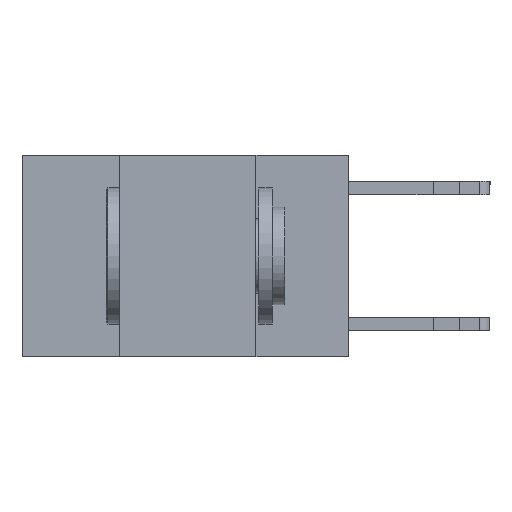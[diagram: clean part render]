
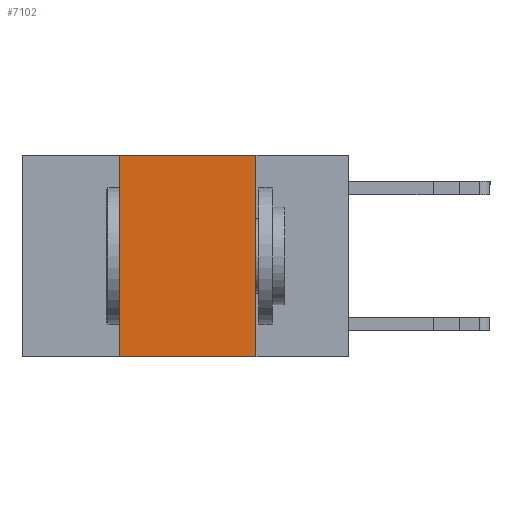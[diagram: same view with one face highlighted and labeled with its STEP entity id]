
A CAD part, left-side view. The second image highlights one B-rep face of the part: STEP entity #7102.
In plain terms, the highlighted planar face has unit normal (-1, 0, 0).
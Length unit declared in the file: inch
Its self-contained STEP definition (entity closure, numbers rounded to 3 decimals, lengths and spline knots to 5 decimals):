
#600 = EDGE_CURVE ( 'NONE', #7114, #12517, #6314, .T. ) ;
#650 = VECTOR ( 'NONE', #9430, 39.37008 ) ;
#1277 = VECTOR ( 'NONE', #7304, 39.37008 ) ;
#1414 = CARTESIAN_POINT ( 'NONE',  ( 0., 0.42, 0. ) ) ;
#1795 = DIRECTION ( 'NONE',  ( 0., 0., -1. ) ) ;
#1915 = DIRECTION ( 'NONE',  ( 0., -1., 0. ) ) ;
#2582 = CARTESIAN_POINT ( 'NONE',  ( 0., 0.17, 0. ) ) ;
#2745 = CARTESIAN_POINT ( 'NONE',  ( 0., 0.6, 0. ) ) ;
#2774 = CARTESIAN_POINT ( 'NONE',  ( 0., 0.17, 0. ) ) ;
#3127 = EDGE_LOOP ( 'NONE', ( #8052, #8882, #10350, #4106 ) ) ;
#3254 = EDGE_CURVE ( 'NONE', #12517, #4693, #7524, .T. ) ;
#3392 = LINE ( 'NONE', #4366, #1277 ) ;
#4106 = ORIENTED_EDGE ( 'NONE', *, *, #6701, .T. ) ;
#4366 = CARTESIAN_POINT ( 'NONE',  ( 0., 0.6, -0.37 ) ) ;
#4643 = CARTESIAN_POINT ( 'NONE',  ( 0., 0.6, 0. ) ) ;
#4693 = VERTEX_POINT ( 'NONE', #2582 ) ;
#4769 = EDGE_CURVE ( 'NONE', #4693, #6601, #11996, .T. ) ;
#5043 = DIRECTION ( 'NONE',  ( 0., 0., 1. ) ) ;
#5673 = CARTESIAN_POINT ( 'NONE',  ( 0., 0.42, -0.37 ) ) ;
#5945 = CARTESIAN_POINT ( 'NONE',  ( 0., 0.42, 0. ) ) ;
#6314 = LINE ( 'NONE', #1414, #8711 ) ;
#6601 = VERTEX_POINT ( 'NONE', #12358 ) ;
#6701 = EDGE_CURVE ( 'NONE', #7114, #6601, #3392, .T. ) ;
#7102 = ADVANCED_FACE ( 'NONE', ( #7598 ), #11309, .F. ) ;
#7114 = VERTEX_POINT ( 'NONE', #5673 ) ;
#7304 = DIRECTION ( 'NONE',  ( 0., -1., 0. ) ) ;
#7524 = LINE ( 'NONE', #4643, #8351 ) ;
#7598 = FACE_OUTER_BOUND ( 'NONE', #3127, .T. ) ;
#8052 = ORIENTED_EDGE ( 'NONE', *, *, #4769, .F. ) ;
#8351 = VECTOR ( 'NONE', #1915, 39.37008 ) ;
#8711 = VECTOR ( 'NONE', #5043, 39.37008 ) ;
#8882 = ORIENTED_EDGE ( 'NONE', *, *, #3254, .F. ) ;
#9430 = DIRECTION ( 'NONE',  ( 0., 0., -1. ) ) ;
#10350 = ORIENTED_EDGE ( 'NONE', *, *, #600, .F. ) ;
#10422 = DIRECTION ( 'NONE',  ( 1., 0., 0. ) ) ;
#11309 = PLANE ( 'NONE',  #12342 ) ;
#11996 = LINE ( 'NONE', #2774, #650 ) ;
#12342 = AXIS2_PLACEMENT_3D ( 'NONE', #2745, #10422, #1795 ) ;
#12358 = CARTESIAN_POINT ( 'NONE',  ( 0., 0.17, -0.37 ) ) ;
#12517 = VERTEX_POINT ( 'NONE', #5945 ) ;
